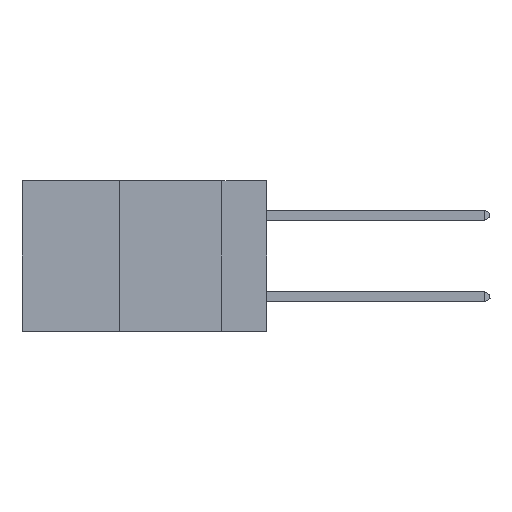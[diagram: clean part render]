
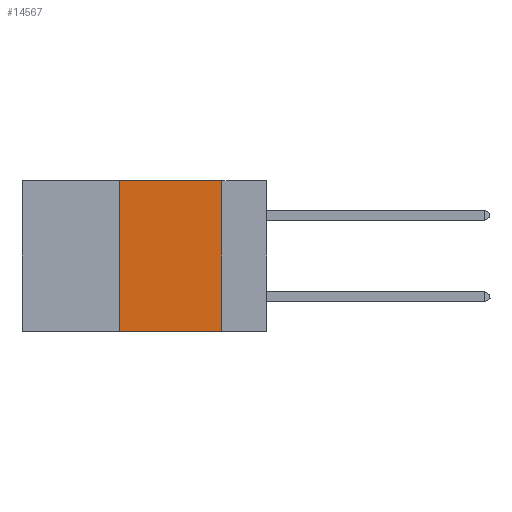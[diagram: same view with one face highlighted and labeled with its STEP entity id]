
A CAD part, left-side view. The second image highlights one B-rep face of the part: STEP entity #14567.
In plain terms, the highlighted planar face has unit normal (-1, 0, 0).
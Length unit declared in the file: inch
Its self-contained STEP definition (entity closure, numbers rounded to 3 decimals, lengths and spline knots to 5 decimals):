
#780 = VERTEX_POINT ( 'NONE', #19782 ) ;
#2242 = DIRECTION ( 'NONE',  ( 0., 0., 1. ) ) ;
#2610 = DIRECTION ( 'NONE',  ( 0., 0., -1. ) ) ;
#2864 = DIRECTION ( 'NONE',  ( 0., -1., 0. ) ) ;
#3722 = PLANE ( 'NONE',  #4017 ) ;
#4017 = AXIS2_PLACEMENT_3D ( 'NONE', #10511, #5557, #19153 ) ;
#4484 = EDGE_CURVE ( 'NONE', #5099, #8582, #9286, .T. ) ;
#4519 = VECTOR ( 'NONE', #2610, 39.37008 ) ;
#5031 = LINE ( 'NONE', #18772, #11388 ) ;
#5099 = VERTEX_POINT ( 'NONE', #10687 ) ;
#5557 = DIRECTION ( 'NONE',  ( 1., 0., 0. ) ) ;
#5623 = EDGE_CURVE ( 'NONE', #780, #8582, #6753, .T. ) ;
#6753 = LINE ( 'NONE', #11874, #16878 ) ;
#7101 = VECTOR ( 'NONE', #2242, 39.37008 ) ;
#8582 = VERTEX_POINT ( 'NONE', #18665 ) ;
#9286 = LINE ( 'NONE', #17409, #4519 ) ;
#9971 = EDGE_CURVE ( 'NONE', #11064, #5099, #5031, .T. ) ;
#10163 = EDGE_CURVE ( 'NONE', #780, #11064, #12157, .T. ) ;
#10511 = CARTESIAN_POINT ( 'NONE',  ( 0., 0.6, 0. ) ) ;
#10687 = CARTESIAN_POINT ( 'NONE',  ( 0., 0.11, 0. ) ) ;
#10706 = ORIENTED_EDGE ( 'NONE', *, *, #10163, .F. ) ;
#11064 = VERTEX_POINT ( 'NONE', #17129 ) ;
#11388 = VECTOR ( 'NONE', #20271, 39.37008 ) ;
#11874 = CARTESIAN_POINT ( 'NONE',  ( 0., 0.6, -0.37 ) ) ;
#12157 = LINE ( 'NONE', #15757, #7101 ) ;
#14567 = ADVANCED_FACE ( 'NONE', ( #21054 ), #3722, .F. ) ;
#15034 = ORIENTED_EDGE ( 'NONE', *, *, #4484, .F. ) ;
#15757 = CARTESIAN_POINT ( 'NONE',  ( 0., 0.36, 0. ) ) ;
#15945 = EDGE_LOOP ( 'NONE', ( #15034, #21183, #10706, #18621 ) ) ;
#16878 = VECTOR ( 'NONE', #2864, 39.37008 ) ;
#17129 = CARTESIAN_POINT ( 'NONE',  ( 0., 0.36, 0. ) ) ;
#17409 = CARTESIAN_POINT ( 'NONE',  ( 0., 0.11, 0. ) ) ;
#18621 = ORIENTED_EDGE ( 'NONE', *, *, #5623, .T. ) ;
#18665 = CARTESIAN_POINT ( 'NONE',  ( 0., 0.11, -0.37 ) ) ;
#18772 = CARTESIAN_POINT ( 'NONE',  ( 0., 0.6, 0. ) ) ;
#19153 = DIRECTION ( 'NONE',  ( 0., 0., -1. ) ) ;
#19782 = CARTESIAN_POINT ( 'NONE',  ( 0., 0.36, -0.37 ) ) ;
#20271 = DIRECTION ( 'NONE',  ( 0., -1., 0. ) ) ;
#21054 = FACE_OUTER_BOUND ( 'NONE', #15945, .T. ) ;
#21183 = ORIENTED_EDGE ( 'NONE', *, *, #9971, .F. ) ;
